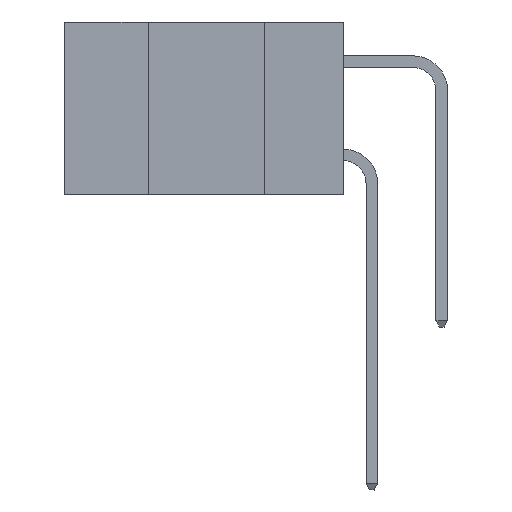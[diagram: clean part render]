
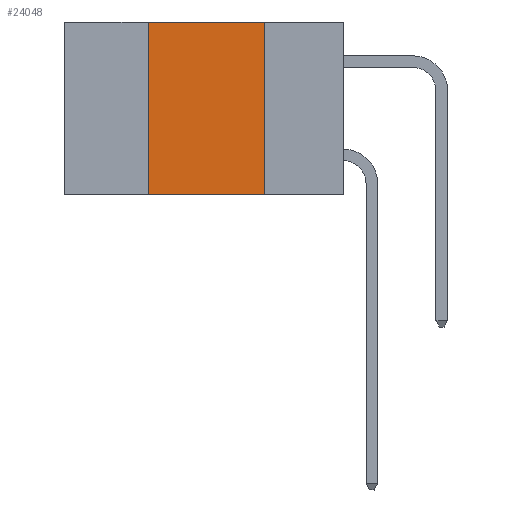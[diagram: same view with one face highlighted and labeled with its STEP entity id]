
A CAD part, left-side view. The second image highlights one B-rep face of the part: STEP entity #24048.
In plain terms, the highlighted planar face has unit normal (-1, 0, 0).
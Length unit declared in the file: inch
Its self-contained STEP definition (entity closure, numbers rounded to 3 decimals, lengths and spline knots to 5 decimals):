
#82 = PLANE ( 'NONE',  #16041 ) ;
#1802 = VERTEX_POINT ( 'NONE', #6146 ) ;
#1887 = DIRECTION ( 'NONE',  ( 1., 0., 0. ) ) ;
#2289 = CARTESIAN_POINT ( 'NONE',  ( 0., 0.17, -0.37 ) ) ;
#2537 = LINE ( 'NONE', #16688, #3285 ) ;
#3018 = VERTEX_POINT ( 'NONE', #3350 ) ;
#3285 = VECTOR ( 'NONE', #27909, 39.37008 ) ;
#3350 = CARTESIAN_POINT ( 'NONE',  ( 0., 0.17, -0.37 ) ) ;
#3420 = EDGE_CURVE ( 'NONE', #5675, #3018, #11360, .T. ) ;
#4650 = VECTOR ( 'NONE', #22896, 39.37008 ) ;
#5675 = VERTEX_POINT ( 'NONE', #29045 ) ;
#5982 = CARTESIAN_POINT ( 'NONE',  ( 0., 0.42, -0.37 ) ) ;
#6146 = CARTESIAN_POINT ( 'NONE',  ( 0., 0.42, 0. ) ) ;
#7703 = LINE ( 'NONE', #16820, #17381 ) ;
#8174 = ORIENTED_EDGE ( 'NONE', *, *, #22553, .F. ) ;
#8718 = DIRECTION ( 'NONE',  ( 0., 0., -1. ) ) ;
#11263 = EDGE_CURVE ( 'NONE', #26201, #3018, #7703, .T. ) ;
#11360 = LINE ( 'NONE', #2289, #4650 ) ;
#13274 = ORIENTED_EDGE ( 'NONE', *, *, #3420, .F. ) ;
#14133 = DIRECTION ( 'NONE',  ( 0., -1., 0. ) ) ;
#14553 = DIRECTION ( 'NONE',  ( 0., -1., 0. ) ) ;
#14841 = LINE ( 'NONE', #21461, #23182 ) ;
#15430 = FACE_OUTER_BOUND ( 'NONE', #19334, .T. ) ;
#16041 = AXIS2_PLACEMENT_3D ( 'NONE', #24887, #1887, #8718 ) ;
#16460 = ORIENTED_EDGE ( 'NONE', *, *, #26259, .F. ) ;
#16688 = CARTESIAN_POINT ( 'NONE',  ( 0., 0.42, -0.37 ) ) ;
#16820 = CARTESIAN_POINT ( 'NONE',  ( 0., 0.6, -0.37 ) ) ;
#17381 = VECTOR ( 'NONE', #14133, 39.37008 ) ;
#19334 = EDGE_LOOP ( 'NONE', ( #13274, #8174, #16460, #23012 ) ) ;
#21461 = CARTESIAN_POINT ( 'NONE',  ( 0., 0.6, 0. ) ) ;
#22553 = EDGE_CURVE ( 'NONE', #1802, #5675, #14841, .T. ) ;
#22896 = DIRECTION ( 'NONE',  ( 0., 0., -1. ) ) ;
#23012 = ORIENTED_EDGE ( 'NONE', *, *, #11263, .T. ) ;
#23182 = VECTOR ( 'NONE', #14553, 39.37008 ) ;
#24048 = ADVANCED_FACE ( 'NONE', ( #15430 ), #82, .F. ) ;
#24887 = CARTESIAN_POINT ( 'NONE',  ( 0., 0.6, 0. ) ) ;
#26201 = VERTEX_POINT ( 'NONE', #5982 ) ;
#26259 = EDGE_CURVE ( 'NONE', #26201, #1802, #2537, .T. ) ;
#27909 = DIRECTION ( 'NONE',  ( 0., 0., 1. ) ) ;
#29045 = CARTESIAN_POINT ( 'NONE',  ( 0., 0.17, 0. ) ) ;
